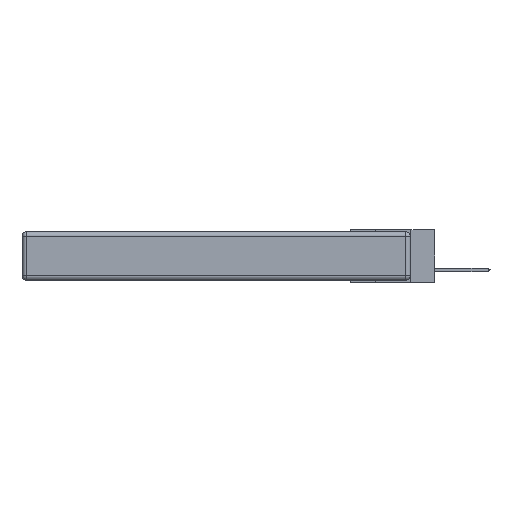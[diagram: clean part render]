
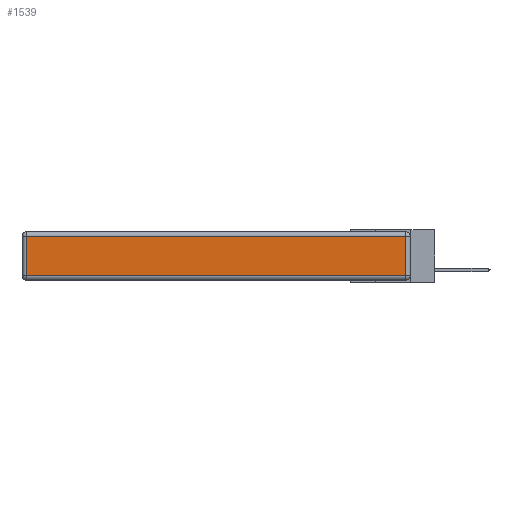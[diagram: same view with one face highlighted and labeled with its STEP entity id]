
A CAD part, left-side view. The second image highlights one B-rep face of the part: STEP entity #1539.
In plain terms, the highlighted planar face has unit normal (-1, 0, 0).
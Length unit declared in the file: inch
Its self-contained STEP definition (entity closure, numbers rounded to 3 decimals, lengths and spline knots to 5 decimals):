
#908 = CARTESIAN_POINT ( 'NONE',  ( 0., 0.03, -0.343 ) ) ;
#1539 = ADVANCED_FACE ( 'NONE', ( #4287 ), #11268, .T. ) ;
#1771 = CARTESIAN_POINT ( 'NONE',  ( 0., 2.72, -0.313 ) ) ;
#2167 = CARTESIAN_POINT ( 'NONE',  ( 0., 0.03, -0.313 ) ) ;
#4287 = FACE_OUTER_BOUND ( 'NONE', #12442, .T. ) ;
#4402 = CARTESIAN_POINT ( 'NONE',  ( 0., 2.75, -0.03 ) ) ;
#4416 = DIRECTION ( 'NONE',  ( 0., 0., 1. ) ) ;
#4948 = LINE ( 'NONE', #908, #29347 ) ;
#6395 = CARTESIAN_POINT ( 'NONE',  ( 0., 0.03, -0.03 ) ) ;
#7990 = LINE ( 'NONE', #30270, #26651 ) ;
#8180 = VERTEX_POINT ( 'NONE', #2167 ) ;
#8565 = ORIENTED_EDGE ( 'NONE', *, *, #13003, .T. ) ;
#9162 = VECTOR ( 'NONE', #22569, 39.37008 ) ;
#11268 = PLANE ( 'NONE',  #28205 ) ;
#12043 = VERTEX_POINT ( 'NONE', #1771 ) ;
#12442 = EDGE_LOOP ( 'NONE', ( #8565, #14663, #31523, #22869 ) ) ;
#12538 = VERTEX_POINT ( 'NONE', #29758 ) ;
#12761 = VECTOR ( 'NONE', #21448, 39.37008 ) ;
#13003 = EDGE_CURVE ( 'NONE', #12043, #8180, #25962, .T. ) ;
#13299 = DIRECTION ( 'NONE',  ( 0., 0., -1. ) ) ;
#13626 = DIRECTION ( 'NONE',  ( 0., 0., 1. ) ) ;
#13796 = EDGE_CURVE ( 'NONE', #8180, #30307, #4948, .T. ) ;
#14663 = ORIENTED_EDGE ( 'NONE', *, *, #13796, .T. ) ;
#17695 = LINE ( 'NONE', #4402, #12761 ) ;
#19018 = CARTESIAN_POINT ( 'NONE',  ( 0., 0., -0.343 ) ) ;
#21448 = DIRECTION ( 'NONE',  ( 0., 1., 0. ) ) ;
#22424 = EDGE_CURVE ( 'NONE', #30307, #12538, #17695, .T. ) ;
#22569 = DIRECTION ( 'NONE',  ( 0., -1., 0. ) ) ;
#22869 = ORIENTED_EDGE ( 'NONE', *, *, #30122, .T. ) ;
#24835 = CARTESIAN_POINT ( 'NONE',  ( 0., 0., -0.313 ) ) ;
#25962 = LINE ( 'NONE', #24835, #9162 ) ;
#26651 = VECTOR ( 'NONE', #13299, 39.37008 ) ;
#28205 = AXIS2_PLACEMENT_3D ( 'NONE', #19018, #30980, #4416 ) ;
#29347 = VECTOR ( 'NONE', #13626, 39.37008 ) ;
#29758 = CARTESIAN_POINT ( 'NONE',  ( 0., 2.72, -0.03 ) ) ;
#30122 = EDGE_CURVE ( 'NONE', #12538, #12043, #7990, .T. ) ;
#30270 = CARTESIAN_POINT ( 'NONE',  ( 0., 2.72, -0.343 ) ) ;
#30307 = VERTEX_POINT ( 'NONE', #6395 ) ;
#30980 = DIRECTION ( 'NONE',  ( -1., 0., 0. ) ) ;
#31523 = ORIENTED_EDGE ( 'NONE', *, *, #22424, .T. ) ;
